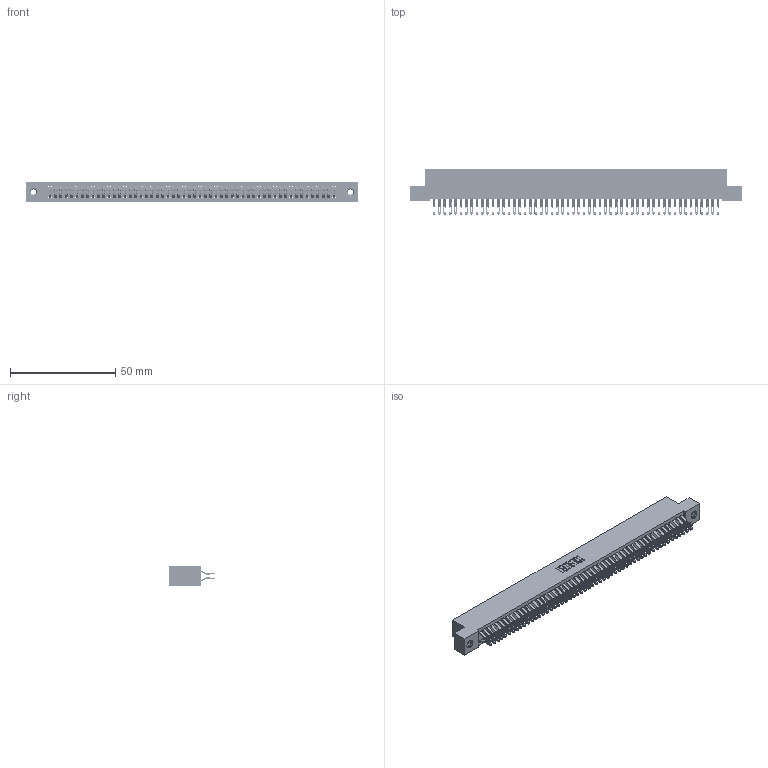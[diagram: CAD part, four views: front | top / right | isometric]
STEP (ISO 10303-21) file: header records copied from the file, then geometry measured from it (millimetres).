
FILE_DESCRIPTION (( 'STEP AP203' ), '1' );
FILE_NAME ('392-108-555-207.STEP', '2018-08-18T21:11:45', ( '' ), ( '' ), 'SwSTEP 2.0', 'SolidWorks 2016', '' );
FILE_SCHEMA (( 'CONFIG_CONTROL_DESIGN' ));
Length unit declared in the file: inch
Products named in the file (4): 345-250-001_345-250-005-103; 392-108-555-207; 342 Part_TI; 345-292-001_555 Tail
Assembly tree (111 placements, depth 2):
  392-108-555-207
    342 Part_TI
    345-292-001_555 Tail  x108
    345-250-001_345-250-005-103  x2
Bounding box: 157.48 x 21.47 x 9.4 mm (x, y, z)
Volume: 14493.8 mm3; surface area: 24958.7 mm2
Topology: 111 solids, 111 shells, 6434 faces, 20199 edges, 13458 vertices
Faces by surface type: plane 3770, cylinder 2648, cone 12, torus 4
Entity records: 34568 total; most frequent: CARTESIAN_POINT 5731, ORIENTED_EDGE 5630, DIRECTION 4877, EDGE_CURVE 2815, LINE 2647, VECTOR 2647, VERTEX_POINT 1872, AXIS2_PLACEMENT_3D 1115
